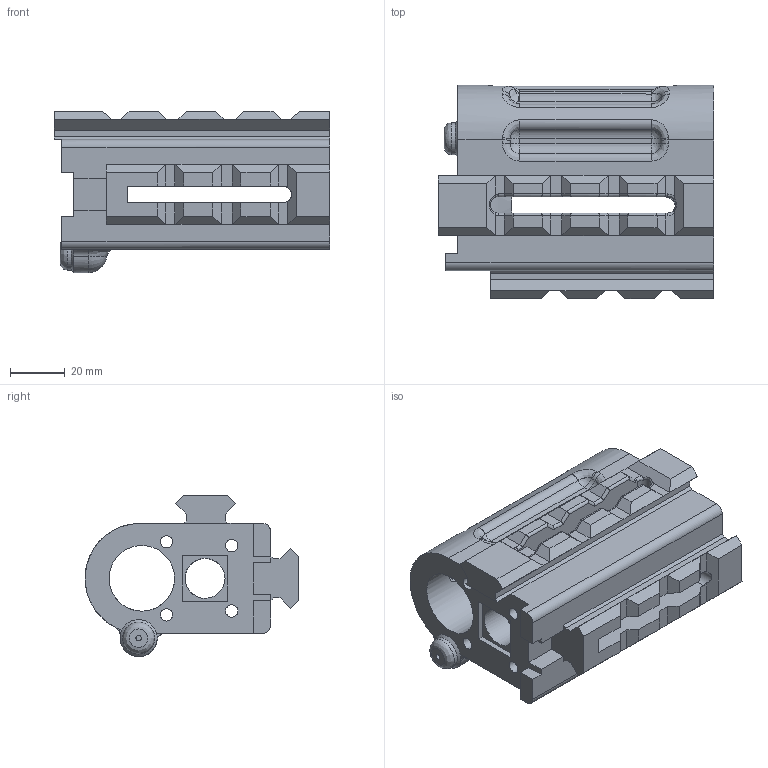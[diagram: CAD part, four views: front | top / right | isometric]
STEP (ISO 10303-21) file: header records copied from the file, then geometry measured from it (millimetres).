
FILE_DESCRIPTION (( 'STEP AP203' ), '1' );
FILE_NAME ('WTF-9_barrel_retainer_grip.STEP', '2020-05-09T09:19:39', ( '' ), ( '' ), 'SwSTEP 2.0', 'SolidWorks 2016', '' );
FILE_SCHEMA (( 'CONFIG_CONTROL_DESIGN' ));
Length unit declared in the file: millimetre
Products named in the file (2): WTF-9_barrel_retainer_grip; WTF9 V1 FINAL_10
Assembly tree (1 placements, depth 2):
  WTF-9_barrel_retainer_grip
    WTF9 V1 FINAL_10
Bounding box: 100.82 x 78.16 x 59.03 mm (x, y, z)
Volume: 154095.3 mm3; surface area: 51222.5 mm2
Topology: 1 solids, 2 shells, 312 faces, 831 edges, 505 vertices
Faces by surface type: plane 138, cylinder 96, bspline 72, torus 5, cone 1
Full cylindrical faces by diameter (mm): 2 x1, 4.5 x4, 11.7 x1, 14.6 x1, 20 x1, 24 x1
Entity records: 14645 total; most frequent: CARTESIAN_POINT 7901, ORIENTED_EDGE 1548, DIRECTION 1037, EDGE_CURVE 774, VERTEX_POINT 475, VECTOR 419, LINE 419, EDGE_LOOP 339
